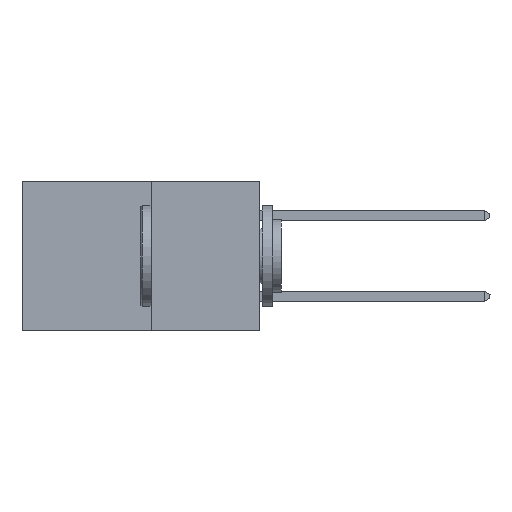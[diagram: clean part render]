
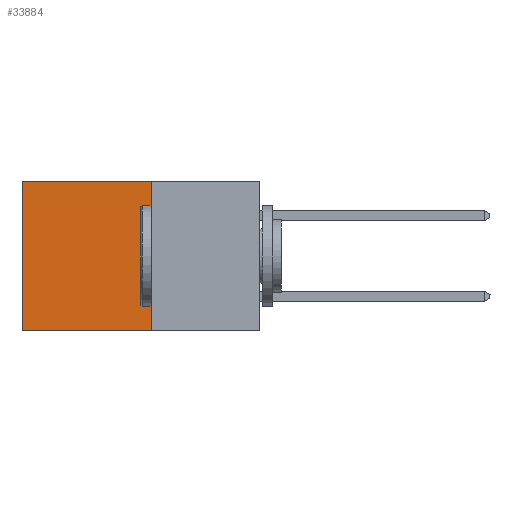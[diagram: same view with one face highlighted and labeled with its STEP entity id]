
A CAD part, left-side view. The second image highlights one B-rep face of the part: STEP entity #33884.
In plain terms, the highlighted planar face has unit normal (-1, 0, 0).
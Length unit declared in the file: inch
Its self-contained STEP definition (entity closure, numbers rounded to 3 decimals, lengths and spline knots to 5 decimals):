
#138 = EDGE_CURVE ( 'NONE', #20215, #19559, #3889, .T. ) ;
#1647 = VECTOR ( 'NONE', #7957, 39.37008 ) ;
#1860 = LINE ( 'NONE', #31143, #30057 ) ;
#3103 = CARTESIAN_POINT ( 'NONE',  ( 0.277, 0.27, -0.37 ) ) ;
#3889 = LINE ( 'NONE', #28819, #23131 ) ;
#4023 = CARTESIAN_POINT ( 'NONE',  ( 0.277, 0.27, -0.37 ) ) ;
#4904 = CARTESIAN_POINT ( 'NONE',  ( 0.277, 0.27, -0.37 ) ) ;
#6806 = DIRECTION ( 'NONE',  ( 0., 0., -1. ) ) ;
#7957 = DIRECTION ( 'NONE',  ( 0., 1., 0. ) ) ;
#8276 = FACE_OUTER_BOUND ( 'NONE', #16744, .T. ) ;
#8847 = VERTEX_POINT ( 'NONE', #11015 ) ;
#10703 = EDGE_CURVE ( 'NONE', #19559, #8847, #1860, .T. ) ;
#11015 = CARTESIAN_POINT ( 'NONE',  ( 0.277, 0.59, -0.37 ) ) ;
#11077 = ORIENTED_EDGE ( 'NONE', *, *, #10703, .T. ) ;
#12108 = ORIENTED_EDGE ( 'NONE', *, *, #138, .T. ) ;
#12756 = AXIS2_PLACEMENT_3D ( 'NONE', #4023, #23140, #6806 ) ;
#14972 = EDGE_CURVE ( 'NONE', #23673, #8847, #16276, .T. ) ;
#16070 = CARTESIAN_POINT ( 'NONE',  ( 0.277, 0.27, -0.37 ) ) ;
#16276 = LINE ( 'NONE', #16070, #1647 ) ;
#16744 = EDGE_LOOP ( 'NONE', ( #11077, #19641, #23400, #12108 ) ) ;
#18526 = EDGE_CURVE ( 'NONE', #20215, #23673, #26371, .T. ) ;
#19145 = VECTOR ( 'NONE', #27705, 39.37008 ) ;
#19559 = VERTEX_POINT ( 'NONE', #20970 ) ;
#19641 = ORIENTED_EDGE ( 'NONE', *, *, #14972, .F. ) ;
#20215 = VERTEX_POINT ( 'NONE', #26282 ) ;
#20896 = DIRECTION ( 'NONE',  ( 0., 1., 0. ) ) ;
#20970 = CARTESIAN_POINT ( 'NONE',  ( 0.277, 0.59, 0. ) ) ;
#23131 = VECTOR ( 'NONE', #20896, 39.37008 ) ;
#23140 = DIRECTION ( 'NONE',  ( 1., 0., 0. ) ) ;
#23400 = ORIENTED_EDGE ( 'NONE', *, *, #18526, .F. ) ;
#23673 = VERTEX_POINT ( 'NONE', #4904 ) ;
#26282 = CARTESIAN_POINT ( 'NONE',  ( 0.277, 0.27, 0. ) ) ;
#26371 = LINE ( 'NONE', #3103, #19145 ) ;
#27705 = DIRECTION ( 'NONE',  ( 0., 0., -1. ) ) ;
#28457 = PLANE ( 'NONE',  #12756 ) ;
#28819 = CARTESIAN_POINT ( 'NONE',  ( 0.277, 0.27, 0. ) ) ;
#30057 = VECTOR ( 'NONE', #33857, 39.37008 ) ;
#31143 = CARTESIAN_POINT ( 'NONE',  ( 0.277, 0.59, -0.37 ) ) ;
#33857 = DIRECTION ( 'NONE',  ( 0., 0., -1. ) ) ;
#33884 = ADVANCED_FACE ( 'NONE', ( #8276 ), #28457, .F. ) ;
